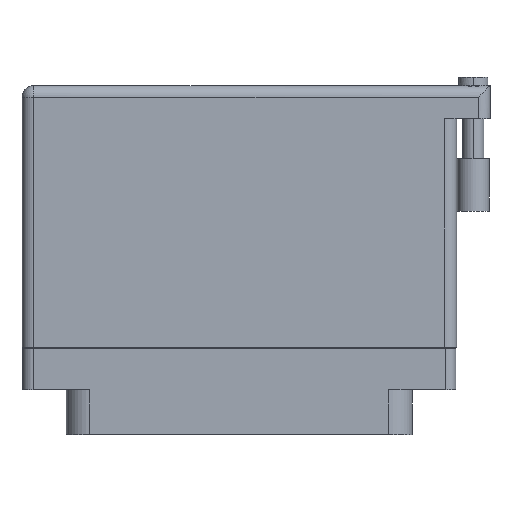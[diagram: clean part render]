
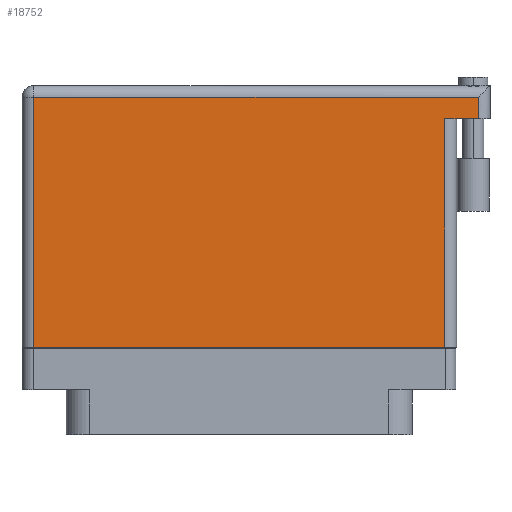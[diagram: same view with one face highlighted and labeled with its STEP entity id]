
A CAD part, front view. The second image highlights one B-rep face of the part: STEP entity #18752.
In plain terms, the highlighted face is planar.
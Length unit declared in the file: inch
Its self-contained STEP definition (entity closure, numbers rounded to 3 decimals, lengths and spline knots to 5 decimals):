
#187 = PLANE ( 'NONE',  #33638 ) ;
#522 = CARTESIAN_POINT ( 'NONE',  ( -1.3, 1.466, 0.4495 ) ) ;
#1953 = CARTESIAN_POINT ( 'NONE',  ( 1.43, 1.466, 0.4495 ) ) ;
#3057 = DIRECTION ( 'NONE',  ( -1., 0., 0. ) ) ;
#3217 = CARTESIAN_POINT ( 'NONE',  ( -1.3, 1.396, 0.4495 ) ) ;
#3336 = CARTESIAN_POINT ( 'NONE',  ( 1.23, -0.1, 0.4495 ) ) ;
#4629 = EDGE_CURVE ( 'NONE', #45240, #5112, #9190, .T. ) ;
#5112 = VERTEX_POINT ( 'NONE', #3336 ) ;
#5693 = DIRECTION ( 'NONE',  ( 0., 1., 0. ) ) ;
#6150 = ORIENTED_EDGE ( 'NONE', *, *, #9945, .F. ) ;
#6590 = CARTESIAN_POINT ( 'NONE',  ( 1.23, 1.269, 0.4495 ) ) ;
#7240 = EDGE_CURVE ( 'NONE', #5112, #43307, #39114, .T. ) ;
#8697 = VECTOR ( 'NONE', #36539, 39.37008 ) ;
#8767 = CARTESIAN_POINT ( 'NONE',  ( 1.5, 1.269, 0.4495 ) ) ;
#9190 = LINE ( 'NONE', #9829, #46985 ) ;
#9829 = CARTESIAN_POINT ( 'NONE',  ( -1.3, -0.1, 0.4495 ) ) ;
#9945 = EDGE_CURVE ( 'NONE', #19362, #43307, #26767, .T. ) ;
#11206 = CARTESIAN_POINT ( 'NONE',  ( -1.23, 1.396, 0.4495 ) ) ;
#12040 = ORIENTED_EDGE ( 'NONE', *, *, #7240, .T. ) ;
#16521 = DIRECTION ( 'NONE',  ( 0., -1., 0. ) ) ;
#17028 = DIRECTION ( 'NONE',  ( 1., 0., 0. ) ) ;
#18752 = ADVANCED_FACE ( 'NONE', ( #42995 ), #187, .F. ) ;
#19362 = VERTEX_POINT ( 'NONE', #37585 ) ;
#19614 = DIRECTION ( 'NONE',  ( -1., 0., 0. ) ) ;
#21246 = CARTESIAN_POINT ( 'NONE',  ( -1.23, -0.1, 0.4495 ) ) ;
#21262 = VERTEX_POINT ( 'NONE', #26156 ) ;
#22109 = DIRECTION ( 'NONE',  ( -1., 0., 0. ) ) ;
#23638 = CARTESIAN_POINT ( 'NONE',  ( -1.23, -0.1, 0.4495 ) ) ;
#23990 = EDGE_LOOP ( 'NONE', ( #46029, #12040, #6150, #33983, #40911, #28864 ) ) ;
#25627 = VECTOR ( 'NONE', #19614, 39.37008 ) ;
#26156 = CARTESIAN_POINT ( 'NONE',  ( 1.43, 1.396, 0.4495 ) ) ;
#26767 = LINE ( 'NONE', #8767, #25627 ) ;
#27348 = EDGE_CURVE ( 'NONE', #19362, #21262, #44183, .T. ) ;
#28470 = LINE ( 'NONE', #3217, #38824 ) ;
#28864 = ORIENTED_EDGE ( 'NONE', *, *, #32641, .T. ) ;
#32641 = EDGE_CURVE ( 'NONE', #33429, #45240, #43113, .T. ) ;
#33429 = VERTEX_POINT ( 'NONE', #11206 ) ;
#33638 = AXIS2_PLACEMENT_3D ( 'NONE', #522, #44030, #22109 ) ;
#33983 = ORIENTED_EDGE ( 'NONE', *, *, #27348, .T. ) ;
#36539 = DIRECTION ( 'NONE',  ( 0., 1., 0. ) ) ;
#36767 = VECTOR ( 'NONE', #5693, 39.37008 ) ;
#37585 = CARTESIAN_POINT ( 'NONE',  ( 1.43, 1.269, 0.4495 ) ) ;
#38824 = VECTOR ( 'NONE', #3057, 39.37008 ) ;
#39114 = LINE ( 'NONE', #44191, #8697 ) ;
#39687 = VECTOR ( 'NONE', #16521, 39.37008 ) ;
#40911 = ORIENTED_EDGE ( 'NONE', *, *, #43341, .T. ) ;
#42995 = FACE_OUTER_BOUND ( 'NONE', #23990, .T. ) ;
#43113 = LINE ( 'NONE', #23638, #39687 ) ;
#43307 = VERTEX_POINT ( 'NONE', #6590 ) ;
#43341 = EDGE_CURVE ( 'NONE', #21262, #33429, #28470, .T. ) ;
#44030 = DIRECTION ( 'NONE',  ( 0., 0., -1. ) ) ;
#44183 = LINE ( 'NONE', #1953, #36767 ) ;
#44191 = CARTESIAN_POINT ( 'NONE',  ( 1.23, 1.269, 0.4495 ) ) ;
#45240 = VERTEX_POINT ( 'NONE', #21246 ) ;
#46029 = ORIENTED_EDGE ( 'NONE', *, *, #4629, .T. ) ;
#46985 = VECTOR ( 'NONE', #17028, 39.37008 ) ;
